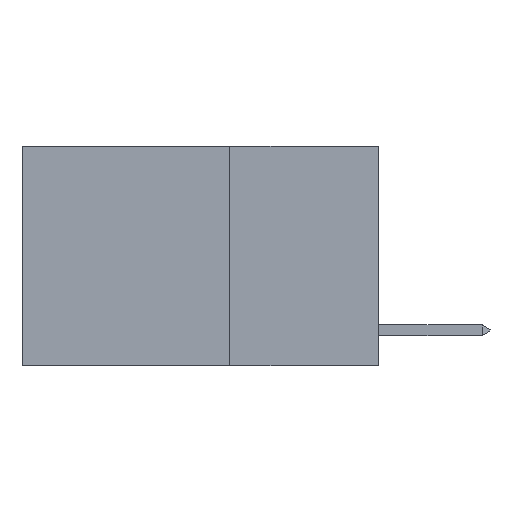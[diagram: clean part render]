
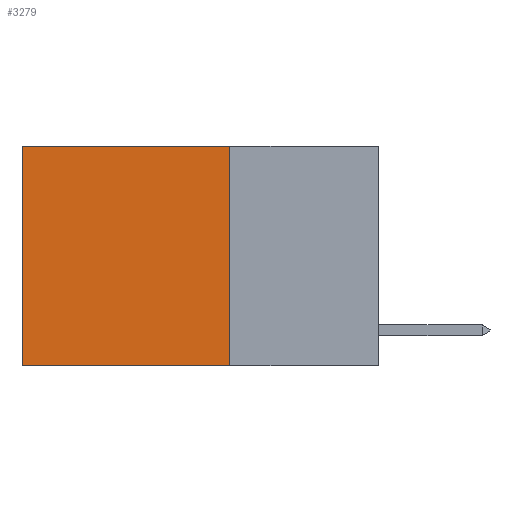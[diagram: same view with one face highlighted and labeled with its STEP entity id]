
A CAD part, left-side view. The second image highlights one B-rep face of the part: STEP entity #3279.
In plain terms, the highlighted planar face has unit normal (-1, 0, 0).
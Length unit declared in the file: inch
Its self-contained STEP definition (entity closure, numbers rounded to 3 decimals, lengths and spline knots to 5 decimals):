
#101 = EDGE_CURVE ( 'NONE', #12145, #5112, #465, .T. ) ;
#154 = ORIENTED_EDGE ( 'NONE', *, *, #101, .F. ) ;
#465 = LINE ( 'NONE', #11491, #17049 ) ;
#1266 = CARTESIAN_POINT ( 'NONE',  ( 0.2625, 0.25, 0. ) ) ;
#1652 = VERTEX_POINT ( 'NONE', #14491 ) ;
#1777 = FACE_OUTER_BOUND ( 'NONE', #6686, .T. ) ;
#1933 = CARTESIAN_POINT ( 'NONE',  ( 0.2625, 0.25, -0.37 ) ) ;
#2695 = LINE ( 'NONE', #15264, #13939 ) ;
#3279 = ADVANCED_FACE ( 'NONE', ( #1777 ), #4386, .F. ) ;
#3331 = DIRECTION ( 'NONE',  ( 0., 1., 0. ) ) ;
#3688 = LINE ( 'NONE', #14703, #16324 ) ;
#4132 = ORIENTED_EDGE ( 'NONE', *, *, #4311, .F. ) ;
#4311 = EDGE_CURVE ( 'NONE', #5112, #15793, #3688, .T. ) ;
#4386 = PLANE ( 'NONE',  #13468 ) ;
#5112 = VERTEX_POINT ( 'NONE', #1933 ) ;
#6677 = ORIENTED_EDGE ( 'NONE', *, *, #8288, .T. ) ;
#6686 = EDGE_LOOP ( 'NONE', ( #6677, #4132, #154, #12771 ) ) ;
#6765 = DIRECTION ( 'NONE',  ( 0., 1., 0. ) ) ;
#6933 = EDGE_CURVE ( 'NONE', #12145, #1652, #8112, .T. ) ;
#8112 = LINE ( 'NONE', #1266, #10439 ) ;
#8209 = DIRECTION ( 'NONE',  ( 0., 0., -1. ) ) ;
#8288 = EDGE_CURVE ( 'NONE', #1652, #15793, #2695, .T. ) ;
#10021 = CARTESIAN_POINT ( 'NONE',  ( 0.2625, 0.25, 0. ) ) ;
#10439 = VECTOR ( 'NONE', #6765, 39.37008 ) ;
#10765 = CARTESIAN_POINT ( 'NONE',  ( 0.2625, 0.25, 0. ) ) ;
#11491 = CARTESIAN_POINT ( 'NONE',  ( 0.2625, 0.25, 0. ) ) ;
#11578 = DIRECTION ( 'NONE',  ( 0., 0., -1. ) ) ;
#12145 = VERTEX_POINT ( 'NONE', #10765 ) ;
#12521 = DIRECTION ( 'NONE',  ( 1., 0., 0. ) ) ;
#12771 = ORIENTED_EDGE ( 'NONE', *, *, #6933, .T. ) ;
#13468 = AXIS2_PLACEMENT_3D ( 'NONE', #10021, #12521, #15342 ) ;
#13939 = VECTOR ( 'NONE', #8209, 39.37008 ) ;
#14491 = CARTESIAN_POINT ( 'NONE',  ( 0.2625, 0.6, 0. ) ) ;
#14703 = CARTESIAN_POINT ( 'NONE',  ( 0.2625, 0.25, -0.37 ) ) ;
#15026 = CARTESIAN_POINT ( 'NONE',  ( 0.2625, 0.6, -0.37 ) ) ;
#15264 = CARTESIAN_POINT ( 'NONE',  ( 0.2625, 0.6, 0. ) ) ;
#15342 = DIRECTION ( 'NONE',  ( 0., 0., -1. ) ) ;
#15793 = VERTEX_POINT ( 'NONE', #15026 ) ;
#16324 = VECTOR ( 'NONE', #3331, 39.37008 ) ;
#17049 = VECTOR ( 'NONE', #11578, 39.37008 ) ;
